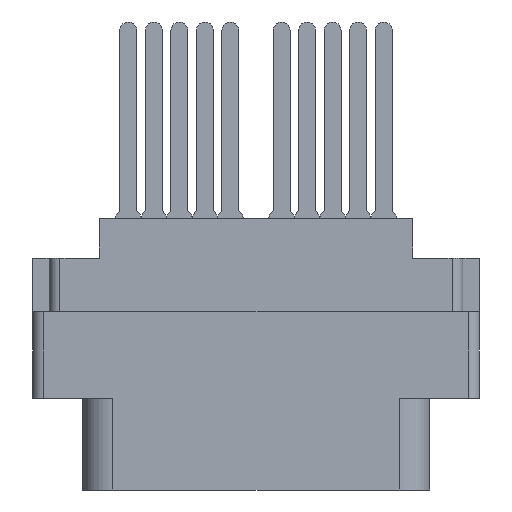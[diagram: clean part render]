
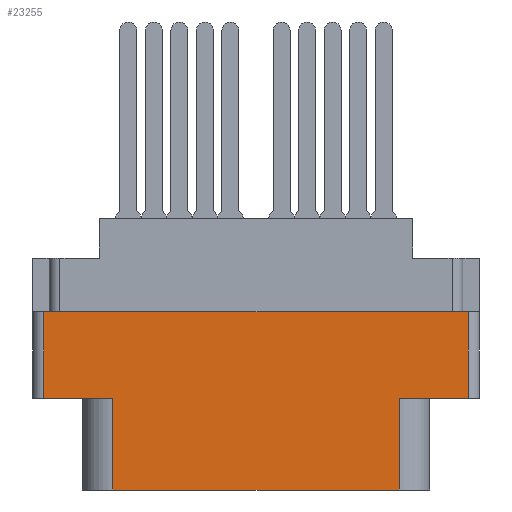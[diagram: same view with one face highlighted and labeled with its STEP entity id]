
A CAD part, front view. The second image highlights one B-rep face of the part: STEP entity #23255.
In plain terms, the highlighted planar face has unit normal (0, -1, 0).
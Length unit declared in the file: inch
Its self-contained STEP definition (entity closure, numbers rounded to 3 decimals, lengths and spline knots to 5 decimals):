
#152 = ORIENTED_EDGE ( 'NONE', *, *, #7861, .T. ) ;
#293 = VERTEX_POINT ( 'NONE', #20109 ) ;
#359 = CARTESIAN_POINT ( 'NONE',  ( -0.624, -0.343, -0.274 ) ) ;
#1153 = ORIENTED_EDGE ( 'NONE', *, *, #12880, .T. ) ;
#1195 = VECTOR ( 'NONE', #8886, 39.37008 ) ;
#1741 = LINE ( 'NONE', #18152, #14178 ) ;
#1981 = DIRECTION ( 'NONE',  ( 0., 0., -1. ) ) ;
#2200 = CARTESIAN_POINT ( 'NONE',  ( -0.42052, -0.343, -0.529 ) ) ;
#3739 = LINE ( 'NONE', #18935, #5740 ) ;
#3740 = VERTEX_POINT ( 'NONE', #2200 ) ;
#3741 = FACE_OUTER_BOUND ( 'NONE', #17156, .T. ) ;
#3749 = EDGE_CURVE ( 'NONE', #6496, #3740, #17258, .T. ) ;
#4652 = VECTOR ( 'NONE', #14614, 39.37008 ) ;
#4806 = ORIENTED_EDGE ( 'NONE', *, *, #7399, .F. ) ;
#5528 = CARTESIAN_POINT ( 'NONE',  ( 0.42052, -0.343, -0.529 ) ) ;
#5740 = VECTOR ( 'NONE', #9959, 39.37008 ) ;
#6496 = VERTEX_POINT ( 'NONE', #20942 ) ;
#6598 = VECTOR ( 'NONE', #15461, 39.37008 ) ;
#6722 = DIRECTION ( 'NONE',  ( 1., 0., 0. ) ) ;
#7399 = EDGE_CURVE ( 'NONE', #18305, #293, #9295, .T. ) ;
#7861 = EDGE_CURVE ( 'NONE', #14465, #293, #16534, .T. ) ;
#8464 = EDGE_CURVE ( 'NONE', #21926, #22624, #1741, .T. ) ;
#8595 = AXIS2_PLACEMENT_3D ( 'NONE', #9549, #22563, #1981 ) ;
#8856 = ORIENTED_EDGE ( 'NONE', *, *, #8464, .T. ) ;
#8886 = DIRECTION ( 'NONE',  ( 0., 0., 1. ) ) ;
#9258 = ORIENTED_EDGE ( 'NONE', *, *, #9871, .T. ) ;
#9295 = LINE ( 'NONE', #18243, #4652 ) ;
#9549 = CARTESIAN_POINT ( 'NONE',  ( -0.656, -0.343, -0.798 ) ) ;
#9871 = EDGE_CURVE ( 'NONE', #15673, #21926, #19207, .T. ) ;
#9959 = DIRECTION ( 'NONE',  ( 0., 0., -1. ) ) ;
#10123 = ORIENTED_EDGE ( 'NONE', *, *, #3749, .T. ) ;
#11423 = VECTOR ( 'NONE', #6722, 39.37008 ) ;
#11784 = CARTESIAN_POINT ( 'NONE',  ( -0.42052, -0.343, -0.798 ) ) ;
#12880 = EDGE_CURVE ( 'NONE', #18305, #6496, #3739, .T. ) ;
#13365 = ORIENTED_EDGE ( 'NONE', *, *, #17276, .F. ) ;
#13433 = DIRECTION ( 'NONE',  ( 1., 0., 0. ) ) ;
#13447 = CARTESIAN_POINT ( 'NONE',  ( -0.42052, -0.343, -0.798 ) ) ;
#14178 = VECTOR ( 'NONE', #21872, 39.37008 ) ;
#14465 = VERTEX_POINT ( 'NONE', #18009 ) ;
#14614 = DIRECTION ( 'NONE',  ( 1., 0., 0. ) ) ;
#15461 = DIRECTION ( 'NONE',  ( 0., 0., -1. ) ) ;
#15486 = ORIENTED_EDGE ( 'NONE', *, *, #23347, .T. ) ;
#15673 = VERTEX_POINT ( 'NONE', #11784 ) ;
#16534 = LINE ( 'NONE', #19921, #1195 ) ;
#17156 = EDGE_LOOP ( 'NONE', ( #4806, #1153, #10123, #15486, #9258, #8856, #13365, #152 ) ) ;
#17258 = LINE ( 'NONE', #22709, #23243 ) ;
#17276 = EDGE_CURVE ( 'NONE', #14465, #22624, #20157, .T. ) ;
#17735 = CARTESIAN_POINT ( 'NONE',  ( -0.656, -0.343, -0.798 ) ) ;
#18009 = CARTESIAN_POINT ( 'NONE',  ( 0.624, -0.343, -0.529 ) ) ;
#18152 = CARTESIAN_POINT ( 'NONE',  ( 0.42052, -0.343, -0.529 ) ) ;
#18243 = CARTESIAN_POINT ( 'NONE',  ( 0., -0.343, -0.274 ) ) ;
#18305 = VERTEX_POINT ( 'NONE', #359 ) ;
#18715 = CARTESIAN_POINT ( 'NONE',  ( 0.42052, -0.343, -0.798 ) ) ;
#18935 = CARTESIAN_POINT ( 'NONE',  ( -0.624, -0.343, -0.798 ) ) ;
#19207 = LINE ( 'NONE', #17735, #11423 ) ;
#19921 = CARTESIAN_POINT ( 'NONE',  ( 0.624, -0.343, -0.798 ) ) ;
#20109 = CARTESIAN_POINT ( 'NONE',  ( 0.624, -0.343, -0.274 ) ) ;
#20157 = LINE ( 'NONE', #23471, #20988 ) ;
#20717 = PLANE ( 'NONE',  #8595 ) ;
#20942 = CARTESIAN_POINT ( 'NONE',  ( -0.624, -0.343, -0.529 ) ) ;
#20988 = VECTOR ( 'NONE', #23221, 39.37008 ) ;
#21872 = DIRECTION ( 'NONE',  ( 0., 0., 1. ) ) ;
#21926 = VERTEX_POINT ( 'NONE', #18715 ) ;
#22155 = LINE ( 'NONE', #13447, #6598 ) ;
#22563 = DIRECTION ( 'NONE',  ( 0., -1., 0. ) ) ;
#22624 = VERTEX_POINT ( 'NONE', #5528 ) ;
#22709 = CARTESIAN_POINT ( 'NONE',  ( 0., -0.343, -0.529 ) ) ;
#23221 = DIRECTION ( 'NONE',  ( -1., 0., 0. ) ) ;
#23243 = VECTOR ( 'NONE', #13433, 39.37008 ) ;
#23255 = ADVANCED_FACE ( 'NONE', ( #3741 ), #20717, .T. ) ;
#23347 = EDGE_CURVE ( 'NONE', #3740, #15673, #22155, .T. ) ;
#23471 = CARTESIAN_POINT ( 'NONE',  ( 0., -0.343, -0.529 ) ) ;
